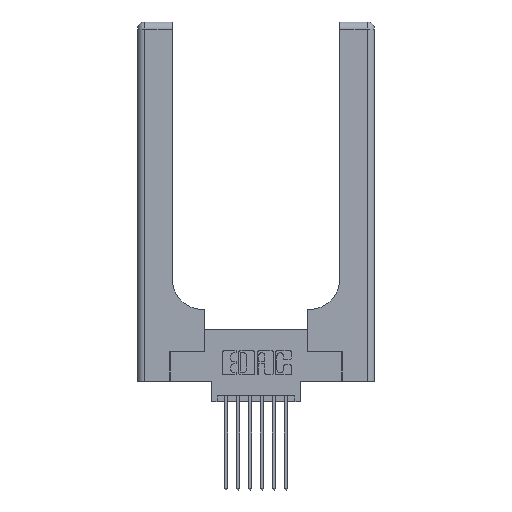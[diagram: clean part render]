
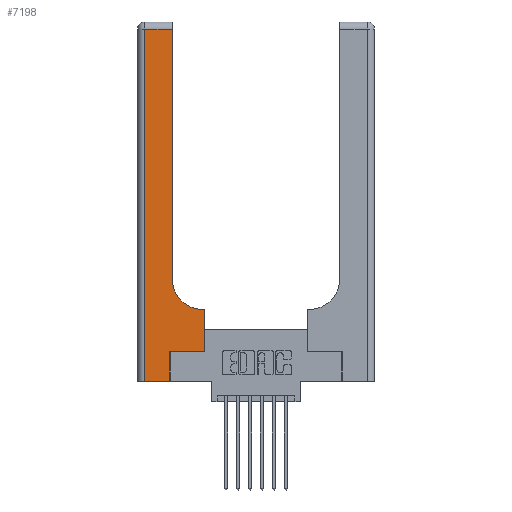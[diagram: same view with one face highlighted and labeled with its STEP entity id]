
A CAD part, top view. The second image highlights one B-rep face of the part: STEP entity #7198.
In plain terms, the highlighted planar face has unit normal (0, 0, 1).
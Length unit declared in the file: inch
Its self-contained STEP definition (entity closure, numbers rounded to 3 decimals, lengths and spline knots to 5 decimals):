
#166 = AXIS2_PLACEMENT_3D ( 'NONE', #2272, #10354, #3478 ) ;
#811 = ORIENTED_EDGE ( 'NONE', *, *, #14705, .T. ) ;
#836 = CARTESIAN_POINT ( 'NONE',  ( 0.5415, 0.85, 0.37 ) ) ;
#899 = ORIENTED_EDGE ( 'NONE', *, *, #5266, .T. ) ;
#1069 = EDGE_CURVE ( 'NONE', #5013, #4989, #5603, .T. ) ;
#1097 = CARTESIAN_POINT ( 'NONE',  ( 0.06, 2.94, 0.37 ) ) ;
#1173 = DIRECTION ( 'NONE',  ( 1., 0., 0. ) ) ;
#1225 = CARTESIAN_POINT ( 'NONE',  ( 0.269, 0.25, 0.37 ) ) ;
#1477 = VERTEX_POINT ( 'NONE', #8029 ) ;
#2032 = DIRECTION ( 'NONE',  ( 1., 0., 0. ) ) ;
#2272 = CARTESIAN_POINT ( 'NONE',  ( 0., 3., 0.37 ) ) ;
#2422 = VERTEX_POINT ( 'NONE', #4059 ) ;
#2627 = CARTESIAN_POINT ( 'NONE',  ( 0.5585, 0.25, 0.37 ) ) ;
#2789 = EDGE_LOOP ( 'NONE', ( #899, #811, #5915, #4547, #5697, #4449, #5364, #5944, #5233 ) ) ;
#2944 = CARTESIAN_POINT ( 'NONE',  ( 0.269, 0., 0.37 ) ) ;
#3190 = VECTOR ( 'NONE', #12486, 39.37008 ) ;
#3478 = DIRECTION ( 'NONE',  ( -1., 0., 0. ) ) ;
#3872 = VECTOR ( 'NONE', #11234, 39.37008 ) ;
#4013 = DIRECTION ( 'NONE',  ( -1., 0., 0. ) ) ;
#4059 = CARTESIAN_POINT ( 'NONE',  ( 0.2915, 2.94, 0.37 ) ) ;
#4150 = AXIS2_PLACEMENT_3D ( 'NONE', #836, #9019, #2032 ) ;
#4234 = FACE_OUTER_BOUND ( 'NONE', #2789, .T. ) ;
#4311 = CIRCLE ( 'NONE', #4150, 0.25 ) ;
#4316 = LINE ( 'NONE', #1225, #10045 ) ;
#4449 = ORIENTED_EDGE ( 'NONE', *, *, #9922, .T. ) ;
#4547 = ORIENTED_EDGE ( 'NONE', *, *, #12659, .T. ) ;
#4660 = EDGE_CURVE ( 'NONE', #1477, #14186, #4311, .T. ) ;
#4989 = VERTEX_POINT ( 'NONE', #5259 ) ;
#5013 = VERTEX_POINT ( 'NONE', #2944 ) ;
#5233 = ORIENTED_EDGE ( 'NONE', *, *, #4660, .T. ) ;
#5259 = CARTESIAN_POINT ( 'NONE',  ( 0.269, 0.25, 0.37 ) ) ;
#5266 = EDGE_CURVE ( 'NONE', #14186, #2422, #6323, .T. ) ;
#5364 = ORIENTED_EDGE ( 'NONE', *, *, #10772, .T. ) ;
#5603 = LINE ( 'NONE', #14804, #13890 ) ;
#5697 = ORIENTED_EDGE ( 'NONE', *, *, #1069, .T. ) ;
#5795 = PLANE ( 'NONE',  #166 ) ;
#5866 = CARTESIAN_POINT ( 'NONE',  ( 0.5585, 0.6, 0.37 ) ) ;
#5915 = ORIENTED_EDGE ( 'NONE', *, *, #8002, .T. ) ;
#5944 = ORIENTED_EDGE ( 'NONE', *, *, #10341, .T. ) ;
#6064 = DIRECTION ( 'NONE',  ( 0., 1., 0. ) ) ;
#6074 = CARTESIAN_POINT ( 'NONE',  ( 0., 0., 0.37 ) ) ;
#6125 = DIRECTION ( 'NONE',  ( 1., 0., 0. ) ) ;
#6323 = LINE ( 'NONE', #10174, #3190 ) ;
#6730 = CARTESIAN_POINT ( 'NONE',  ( 0.06, 3., 0.37 ) ) ;
#7088 = VERTEX_POINT ( 'NONE', #12389 ) ;
#7142 = LINE ( 'NONE', #6730, #3872 ) ;
#7198 = ADVANCED_FACE ( 'NONE', ( #4234 ), #5795, .F. ) ;
#7658 = DIRECTION ( 'NONE',  ( 0., 1., 0. ) ) ;
#7862 = LINE ( 'NONE', #7992, #13098 ) ;
#7992 = CARTESIAN_POINT ( 'NONE',  ( 0., 2.94, 0.37 ) ) ;
#8002 = EDGE_CURVE ( 'NONE', #11655, #7088, #7142, .T. ) ;
#8029 = CARTESIAN_POINT ( 'NONE',  ( 0.5415, 0.6, 0.37 ) ) ;
#8134 = CARTESIAN_POINT ( 'NONE',  ( 0.2915, 0.85, 0.37 ) ) ;
#8617 = CARTESIAN_POINT ( 'NONE',  ( 0.2915, 0.6, 0.37 ) ) ;
#8650 = VECTOR ( 'NONE', #6064, 39.37008 ) ;
#9019 = DIRECTION ( 'NONE',  ( 0., 0., -1. ) ) ;
#9632 = LINE ( 'NONE', #6074, #12625 ) ;
#9922 = EDGE_CURVE ( 'NONE', #4989, #10239, #4316, .T. ) ;
#10045 = VECTOR ( 'NONE', #1173, 39.37008 ) ;
#10174 = CARTESIAN_POINT ( 'NONE',  ( 0.2915, 3., 0.37 ) ) ;
#10239 = VERTEX_POINT ( 'NONE', #2627 ) ;
#10341 = EDGE_CURVE ( 'NONE', #13686, #1477, #13902, .T. ) ;
#10354 = DIRECTION ( 'NONE',  ( 0., 0., -1. ) ) ;
#10772 = EDGE_CURVE ( 'NONE', #10239, #13686, #11619, .T. ) ;
#10931 = VECTOR ( 'NONE', #4013, 39.37008 ) ;
#11234 = DIRECTION ( 'NONE',  ( 0., -1., 0. ) ) ;
#11326 = DIRECTION ( 'NONE',  ( -1., 0., 0. ) ) ;
#11619 = LINE ( 'NONE', #11685, #8650 ) ;
#11655 = VERTEX_POINT ( 'NONE', #1097 ) ;
#11685 = CARTESIAN_POINT ( 'NONE',  ( 0.5585, 0.25, 0.37 ) ) ;
#12389 = CARTESIAN_POINT ( 'NONE',  ( 0.06, 0., 0.37 ) ) ;
#12486 = DIRECTION ( 'NONE',  ( 0., 1., 0. ) ) ;
#12625 = VECTOR ( 'NONE', #6125, 39.37008 ) ;
#12659 = EDGE_CURVE ( 'NONE', #7088, #5013, #9632, .T. ) ;
#13098 = VECTOR ( 'NONE', #11326, 39.37008 ) ;
#13686 = VERTEX_POINT ( 'NONE', #5866 ) ;
#13890 = VECTOR ( 'NONE', #7658, 39.37008 ) ;
#13902 = LINE ( 'NONE', #8617, #10931 ) ;
#14186 = VERTEX_POINT ( 'NONE', #8134 ) ;
#14705 = EDGE_CURVE ( 'NONE', #2422, #11655, #7862, .T. ) ;
#14804 = CARTESIAN_POINT ( 'NONE',  ( 0.269, 0., 0.37 ) ) ;
